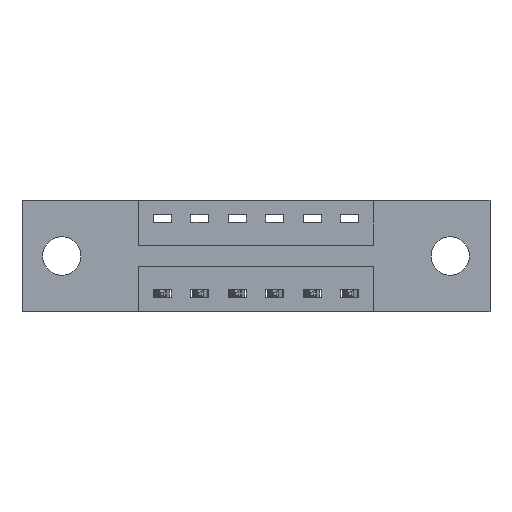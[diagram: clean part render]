
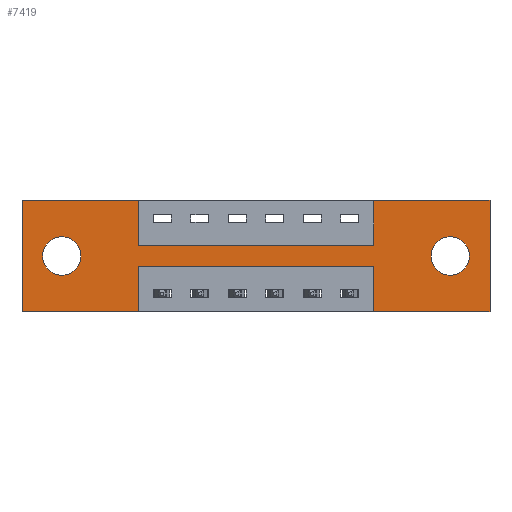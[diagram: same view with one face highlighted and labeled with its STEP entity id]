
A CAD part, front view. The second image highlights one B-rep face of the part: STEP entity #7419.
In plain terms, the highlighted planar face has unit normal (0, -1, 0).
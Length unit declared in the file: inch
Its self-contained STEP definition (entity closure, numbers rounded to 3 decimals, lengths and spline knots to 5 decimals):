
#21 = DIRECTION ( 'NONE',  ( 0., 0., 1. ) ) ;
#146 = CARTESIAN_POINT ( 'NONE',  ( 0.3875, 0., -0.22 ) ) ;
#317 = ORIENTED_EDGE ( 'NONE', *, *, #7982, .F. ) ;
#343 = EDGE_CURVE ( 'NONE', #4749, #1883, #6066, .T. ) ;
#424 = CARTESIAN_POINT ( 'NONE',  ( 0.1325, 0., -0.185 ) ) ;
#449 = CARTESIAN_POINT ( 'NONE',  ( 0.1325, 0., -0.185 ) ) ;
#458 = LINE ( 'NONE', #5784, #7281 ) ;
#486 = EDGE_CURVE ( 'NONE', #6126, #6779, #6733, .T. ) ;
#490 = ORIENTED_EDGE ( 'NONE', *, *, #1294, .F. ) ;
#538 = CARTESIAN_POINT ( 'NONE',  ( 1.4275, 0., -0.121 ) ) ;
#581 = DIRECTION ( 'NONE',  ( 0., -1., 0. ) ) ;
#595 = EDGE_CURVE ( 'NONE', #5809, #5454, #6927, .T. ) ;
#753 = EDGE_CURVE ( 'NONE', #1500, #5809, #3041, .T. ) ;
#759 = ORIENTED_EDGE ( 'NONE', *, *, #753, .F. ) ;
#795 = CARTESIAN_POINT ( 'NONE',  ( 1.4275, 0., -0.185 ) ) ;
#811 = CIRCLE ( 'NONE', #2363, 0.064 ) ;
#978 = ORIENTED_EDGE ( 'NONE', *, *, #2827, .F. ) ;
#1074 = DIRECTION ( 'NONE',  ( 0., 0., 1. ) ) ;
#1111 = CARTESIAN_POINT ( 'NONE',  ( 1.56, 0., 0. ) ) ;
#1237 = FACE_OUTER_BOUND ( 'NONE', #3675, .T. ) ;
#1271 = CARTESIAN_POINT ( 'NONE',  ( 0.3875, 0., -0.15 ) ) ;
#1294 = EDGE_CURVE ( 'NONE', #6889, #8308, #458, .T. ) ;
#1500 = VERTEX_POINT ( 'NONE', #7145 ) ;
#1589 = LINE ( 'NONE', #4819, #2843 ) ;
#1667 = EDGE_CURVE ( 'NONE', #6724, #7783, #4698, .T. ) ;
#1703 = LINE ( 'NONE', #7011, #2127 ) ;
#1736 = DIRECTION ( 'NONE',  ( 1., 0., 0. ) ) ;
#1836 = DIRECTION ( 'NONE',  ( 0., 0., -1. ) ) ;
#1866 = CARTESIAN_POINT ( 'NONE',  ( 0.3875, 0., -0.15 ) ) ;
#1883 = VERTEX_POINT ( 'NONE', #4702 ) ;
#1954 = ORIENTED_EDGE ( 'NONE', *, *, #4395, .F. ) ;
#2018 = ORIENTED_EDGE ( 'NONE', *, *, #4690, .F. ) ;
#2065 = CARTESIAN_POINT ( 'NONE',  ( 0., 0., 0. ) ) ;
#2127 = VECTOR ( 'NONE', #1836, 39.37008 ) ;
#2141 = CARTESIAN_POINT ( 'NONE',  ( 0., 0., -0.37 ) ) ;
#2163 = DIRECTION ( 'NONE',  ( 0., 1., 0. ) ) ;
#2195 = CARTESIAN_POINT ( 'NONE',  ( 1.1725, 0., 0. ) ) ;
#2249 = ORIENTED_EDGE ( 'NONE', *, *, #486, .T. ) ;
#2363 = AXIS2_PLACEMENT_3D ( 'NONE', #449, #3772, #3683 ) ;
#2448 = EDGE_LOOP ( 'NONE', ( #2249, #4623 ) ) ;
#2492 = DIRECTION ( 'NONE',  ( 0., 1., 0. ) ) ;
#2551 = CARTESIAN_POINT ( 'NONE',  ( 1.1725, 0., -0.37 ) ) ;
#2800 = CARTESIAN_POINT ( 'NONE',  ( 1.1725, 0., -0.15 ) ) ;
#2822 = CARTESIAN_POINT ( 'NONE',  ( 0.1325, 0., -0.121 ) ) ;
#2827 = EDGE_CURVE ( 'NONE', #1883, #3725, #1703, .T. ) ;
#2843 = VECTOR ( 'NONE', #7513, 39.37008 ) ;
#2848 = ORIENTED_EDGE ( 'NONE', *, *, #3643, .T. ) ;
#2873 = CARTESIAN_POINT ( 'NONE',  ( 1.4275, 0., -0.185 ) ) ;
#2885 = CARTESIAN_POINT ( 'NONE',  ( 0.3875, 0., -0.22 ) ) ;
#2901 = VECTOR ( 'NONE', #21, 39.37008 ) ;
#2982 = AXIS2_PLACEMENT_3D ( 'NONE', #2873, #8217, #4224 ) ;
#3041 = LINE ( 'NONE', #1111, #6744 ) ;
#3092 = DIRECTION ( 'NONE',  ( -1., 0., 0. ) ) ;
#3099 = VECTOR ( 'NONE', #8210, 39.37008 ) ;
#3173 = VECTOR ( 'NONE', #3482, 39.37008 ) ;
#3269 = EDGE_CURVE ( 'NONE', #3725, #6724, #7701, .T. ) ;
#3314 = LINE ( 'NONE', #8055, #3173 ) ;
#3321 = VECTOR ( 'NONE', #4156, 39.37008 ) ;
#3471 = DIRECTION ( 'NONE',  ( 0., 0., -1. ) ) ;
#3482 = DIRECTION ( 'NONE',  ( 1., 0., 0. ) ) ;
#3502 = DIRECTION ( 'NONE',  ( 1., 0., 0. ) ) ;
#3518 = ORIENTED_EDGE ( 'NONE', *, *, #7022, .T. ) ;
#3555 = CARTESIAN_POINT ( 'NONE',  ( 0.3875, 0., -0.37 ) ) ;
#3594 = AXIS2_PLACEMENT_3D ( 'NONE', #3810, #581, #8384 ) ;
#3643 = EDGE_CURVE ( 'NONE', #5798, #4735, #811, .T. ) ;
#3667 = VERTEX_POINT ( 'NONE', #5773 ) ;
#3675 = EDGE_LOOP ( 'NONE', ( #1954, #317, #2018, #4382, #759, #5410, #6135, #4678, #978, #5063, #4176, #490 ) ) ;
#3683 = DIRECTION ( 'NONE',  ( 0., 0., 1. ) ) ;
#3725 = VERTEX_POINT ( 'NONE', #1271 ) ;
#3771 = VECTOR ( 'NONE', #1736, 39.37008 ) ;
#3772 = DIRECTION ( 'NONE',  ( 0., 1., 0. ) ) ;
#3810 = CARTESIAN_POINT ( 'NONE',  ( 0., 0., -0.37 ) ) ;
#4156 = DIRECTION ( 'NONE',  ( -1., 0., 0. ) ) ;
#4176 = ORIENTED_EDGE ( 'NONE', *, *, #4953, .F. ) ;
#4212 = LINE ( 'NONE', #3555, #3099 ) ;
#4224 = DIRECTION ( 'NONE',  ( 0., 0., -1. ) ) ;
#4382 = ORIENTED_EDGE ( 'NONE', *, *, #595, .F. ) ;
#4395 = EDGE_CURVE ( 'NONE', #8584, #6889, #4212, .T. ) ;
#4484 = FACE_BOUND ( 'NONE', #2448, .T. ) ;
#4623 = ORIENTED_EDGE ( 'NONE', *, *, #8015, .T. ) ;
#4678 = ORIENTED_EDGE ( 'NONE', *, *, #3269, .F. ) ;
#4690 = EDGE_CURVE ( 'NONE', #5454, #3667, #1589, .T. ) ;
#4698 = LINE ( 'NONE', #5298, #2901 ) ;
#4702 = CARTESIAN_POINT ( 'NONE',  ( 0.3875, 0., 0. ) ) ;
#4735 = VERTEX_POINT ( 'NONE', #2822 ) ;
#4749 = VERTEX_POINT ( 'NONE', #5461 ) ;
#4819 = CARTESIAN_POINT ( 'NONE',  ( 1.1725, 0., -0.37 ) ) ;
#4953 = EDGE_CURVE ( 'NONE', #8308, #4749, #6599, .T. ) ;
#5063 = ORIENTED_EDGE ( 'NONE', *, *, #343, .F. ) ;
#5204 = FACE_BOUND ( 'NONE', #6371, .T. ) ;
#5298 = CARTESIAN_POINT ( 'NONE',  ( 1.1725, 0., 0. ) ) ;
#5386 = AXIS2_PLACEMENT_3D ( 'NONE', #424, #2492, #1074 ) ;
#5403 = CIRCLE ( 'NONE', #6522, 0.064 ) ;
#5410 = ORIENTED_EDGE ( 'NONE', *, *, #6720, .F. ) ;
#5454 = VERTEX_POINT ( 'NONE', #2551 ) ;
#5461 = CARTESIAN_POINT ( 'NONE',  ( 0., 0., 0. ) ) ;
#5772 = VECTOR ( 'NONE', #7020, 39.37008 ) ;
#5773 = CARTESIAN_POINT ( 'NONE',  ( 1.1725, 0., -0.22 ) ) ;
#5784 = CARTESIAN_POINT ( 'NONE',  ( 0., 0., -0.37 ) ) ;
#5798 = VERTEX_POINT ( 'NONE', #7870 ) ;
#5809 = VERTEX_POINT ( 'NONE', #7575 ) ;
#6066 = LINE ( 'NONE', #7509, #7012 ) ;
#6126 = VERTEX_POINT ( 'NONE', #538 ) ;
#6135 = ORIENTED_EDGE ( 'NONE', *, *, #1667, .F. ) ;
#6366 = CARTESIAN_POINT ( 'NONE',  ( 0.3875, 0., -0.37 ) ) ;
#6371 = EDGE_LOOP ( 'NONE', ( #3518, #2848 ) ) ;
#6522 = AXIS2_PLACEMENT_3D ( 'NONE', #795, #2163, #3471 ) ;
#6599 = LINE ( 'NONE', #2065, #6999 ) ;
#6695 = DIRECTION ( 'NONE',  ( 0., 0., 1. ) ) ;
#6720 = EDGE_CURVE ( 'NONE', #7783, #1500, #3314, .T. ) ;
#6724 = VERTEX_POINT ( 'NONE', #2800 ) ;
#6733 = CIRCLE ( 'NONE', #2982, 0.064 ) ;
#6744 = VECTOR ( 'NONE', #7821, 39.37008 ) ;
#6747 = CARTESIAN_POINT ( 'NONE',  ( 1.4275, 0., -0.249 ) ) ;
#6779 = VERTEX_POINT ( 'NONE', #6747 ) ;
#6889 = VERTEX_POINT ( 'NONE', #6366 ) ;
#6914 = CIRCLE ( 'NONE', #5386, 0.064 ) ;
#6927 = LINE ( 'NONE', #7537, #5772 ) ;
#6948 = LINE ( 'NONE', #146, #3321 ) ;
#6999 = VECTOR ( 'NONE', #6695, 39.37008 ) ;
#7011 = CARTESIAN_POINT ( 'NONE',  ( 0.3875, 0., 0. ) ) ;
#7012 = VECTOR ( 'NONE', #3502, 39.37008 ) ;
#7020 = DIRECTION ( 'NONE',  ( -1., 0., 0. ) ) ;
#7022 = EDGE_CURVE ( 'NONE', #4735, #5798, #6914, .T. ) ;
#7145 = CARTESIAN_POINT ( 'NONE',  ( 1.56, 0., 0. ) ) ;
#7281 = VECTOR ( 'NONE', #3092, 39.37008 ) ;
#7419 = ADVANCED_FACE ( 'NONE', ( #4484, #5204, #1237 ), #7699, .T. ) ;
#7509 = CARTESIAN_POINT ( 'NONE',  ( 0., 0., 0. ) ) ;
#7513 = DIRECTION ( 'NONE',  ( 0., 0., 1. ) ) ;
#7537 = CARTESIAN_POINT ( 'NONE',  ( 0., 0., -0.37 ) ) ;
#7575 = CARTESIAN_POINT ( 'NONE',  ( 1.56, 0., -0.37 ) ) ;
#7699 = PLANE ( 'NONE',  #3594 ) ;
#7701 = LINE ( 'NONE', #1866, #3771 ) ;
#7783 = VERTEX_POINT ( 'NONE', #2195 ) ;
#7821 = DIRECTION ( 'NONE',  ( 0., 0., -1. ) ) ;
#7870 = CARTESIAN_POINT ( 'NONE',  ( 0.1325, 0., -0.249 ) ) ;
#7982 = EDGE_CURVE ( 'NONE', #3667, #8584, #6948, .T. ) ;
#8015 = EDGE_CURVE ( 'NONE', #6779, #6126, #5403, .T. ) ;
#8055 = CARTESIAN_POINT ( 'NONE',  ( 0., 0., 0. ) ) ;
#8210 = DIRECTION ( 'NONE',  ( 0., 0., -1. ) ) ;
#8217 = DIRECTION ( 'NONE',  ( 0., 1., 0. ) ) ;
#8308 = VERTEX_POINT ( 'NONE', #2141 ) ;
#8384 = DIRECTION ( 'NONE',  ( 0., 0., -1. ) ) ;
#8584 = VERTEX_POINT ( 'NONE', #2885 ) ;
